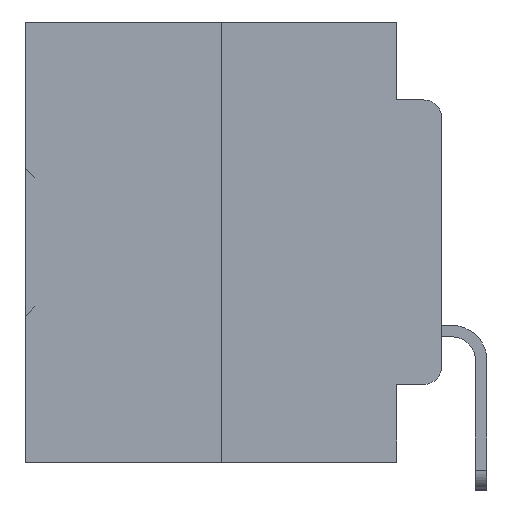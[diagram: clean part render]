
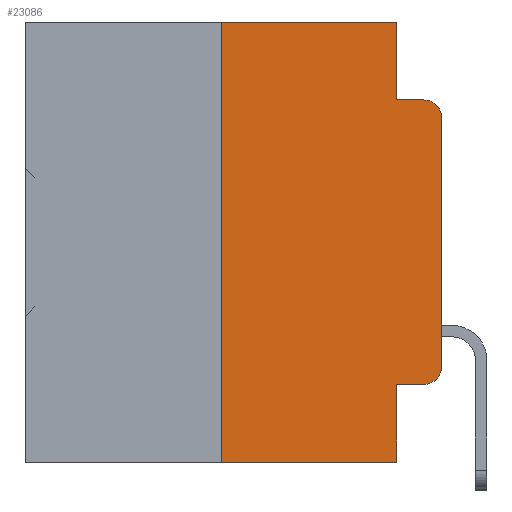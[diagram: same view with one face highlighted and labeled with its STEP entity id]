
A CAD part, left-side view. The second image highlights one B-rep face of the part: STEP entity #23086.
In plain terms, the highlighted planar face has unit normal (-1, 0, 0).
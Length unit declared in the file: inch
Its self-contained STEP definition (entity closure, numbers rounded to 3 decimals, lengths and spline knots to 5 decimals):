
#626 = DIRECTION ( 'NONE',  ( 0., 0., -1. ) ) ;
#1160 = CARTESIAN_POINT ( 'NONE',  ( 0., 0.051, -0.0885 ) ) ;
#1191 = DIRECTION ( 'NONE',  ( 0., -1., 0. ) ) ;
#1412 = ORIENTED_EDGE ( 'NONE', *, *, #22082, .F. ) ;
#1451 = ORIENTED_EDGE ( 'NONE', *, *, #6704, .T. ) ;
#1999 = ORIENTED_EDGE ( 'NONE', *, *, #4632, .T. ) ;
#2195 = ORIENTED_EDGE ( 'NONE', *, *, #2540, .F. ) ;
#2540 = EDGE_CURVE ( 'NONE', #16246, #21346, #27985, .T. ) ;
#3675 = VECTOR ( 'NONE', #13555, 39.37008 ) ;
#4481 = VECTOR ( 'NONE', #35738, 39.37008 ) ;
#4632 = EDGE_CURVE ( 'NONE', #16246, #25232, #21026, .T. ) ;
#5987 = CARTESIAN_POINT ( 'NONE',  ( 0., 0.051, -0.0885 ) ) ;
#6345 = ORIENTED_EDGE ( 'NONE', *, *, #34765, .F. ) ;
#6704 = EDGE_CURVE ( 'NONE', #25232, #14357, #8270, .T. ) ;
#8270 = CIRCLE ( 'NONE', #35639, 0.02 ) ;
#8924 = CARTESIAN_POINT ( 'NONE',  ( 0., 0.25, 0. ) ) ;
#9318 = AXIS2_PLACEMENT_3D ( 'NONE', #10441, #10568, #30804 ) ;
#9824 = CARTESIAN_POINT ( 'NONE',  ( 0., 0., -0.3915 ) ) ;
#10441 = CARTESIAN_POINT ( 'NONE',  ( 0., 0.473, 0. ) ) ;
#10568 = DIRECTION ( 'NONE',  ( 1., 0., 0. ) ) ;
#10607 = VERTEX_POINT ( 'NONE', #23813 ) ;
#10958 = LINE ( 'NONE', #8924, #32226 ) ;
#11064 = LINE ( 'NONE', #36434, #24773 ) ;
#11649 = ORIENTED_EDGE ( 'NONE', *, *, #23069, .T. ) ;
#11837 = LINE ( 'NONE', #1160, #3675 ) ;
#11962 = DIRECTION ( 'NONE',  ( 0., -1., 0. ) ) ;
#12169 = CARTESIAN_POINT ( 'NONE',  ( 0., 0.473, 0. ) ) ;
#13006 = VECTOR ( 'NONE', #626, 39.37008 ) ;
#13555 = DIRECTION ( 'NONE',  ( 0., -1., 0. ) ) ;
#13942 = CARTESIAN_POINT ( 'NONE',  ( 0., 0.051, -0.4115 ) ) ;
#13976 = ORIENTED_EDGE ( 'NONE', *, *, #21432, .T. ) ;
#14116 = ORIENTED_EDGE ( 'NONE', *, *, #25229, .F. ) ;
#14357 = VERTEX_POINT ( 'NONE', #9824 ) ;
#14904 = CIRCLE ( 'NONE', #19058, 0.02 ) ;
#15315 = VECTOR ( 'NONE', #21055, 39.37008 ) ;
#15447 = DIRECTION ( 'NONE',  ( -1., 0., 0. ) ) ;
#16090 = CARTESIAN_POINT ( 'NONE',  ( 0., 0.25, -0.5 ) ) ;
#16244 = LINE ( 'NONE', #12169, #15315 ) ;
#16246 = VERTEX_POINT ( 'NONE', #13942 ) ;
#16647 = ORIENTED_EDGE ( 'NONE', *, *, #19540, .T. ) ;
#17159 = FACE_OUTER_BOUND ( 'NONE', #35326, .T. ) ;
#17378 = ORIENTED_EDGE ( 'NONE', *, *, #32853, .F. ) ;
#17416 = CARTESIAN_POINT ( 'NONE',  ( 0., 0.02, -0.0885 ) ) ;
#17873 = CARTESIAN_POINT ( 'NONE',  ( 0., 0.25, 0. ) ) ;
#18340 = CARTESIAN_POINT ( 'NONE',  ( 0., 0.02, -0.1085 ) ) ;
#19058 = AXIS2_PLACEMENT_3D ( 'NONE', #18340, #37936, #21225 ) ;
#19540 = EDGE_CURVE ( 'NONE', #14357, #10607, #35267, .T. ) ;
#20838 = LINE ( 'NONE', #33101, #13006 ) ;
#21026 = LINE ( 'NONE', #32145, #27666 ) ;
#21055 = DIRECTION ( 'NONE',  ( 0., -1., 0. ) ) ;
#21064 = VECTOR ( 'NONE', #26533, 39.37008 ) ;
#21225 = DIRECTION ( 'NONE',  ( 0., 0., -1. ) ) ;
#21346 = VERTEX_POINT ( 'NONE', #23585 ) ;
#21432 = EDGE_CURVE ( 'NONE', #10607, #27929, #14904, .T. ) ;
#22082 = EDGE_CURVE ( 'NONE', #28594, #37106, #16244, .T. ) ;
#23069 = EDGE_CURVE ( 'NONE', #32886, #21346, #11064, .T. ) ;
#23086 = ADVANCED_FACE ( 'NONE', ( #17159 ), #27964, .F. ) ;
#23585 = CARTESIAN_POINT ( 'NONE',  ( 0., 0.051, -0.5 ) ) ;
#23696 = CARTESIAN_POINT ( 'NONE',  ( 0., 0., 0. ) ) ;
#23813 = CARTESIAN_POINT ( 'NONE',  ( 0., 0., -0.1085 ) ) ;
#24773 = VECTOR ( 'NONE', #1191, 39.37008 ) ;
#25229 = EDGE_CURVE ( 'NONE', #30576, #27929, #11837, .T. ) ;
#25232 = VERTEX_POINT ( 'NONE', #27943 ) ;
#26533 = DIRECTION ( 'NONE',  ( 0., 0., 1. ) ) ;
#27666 = VECTOR ( 'NONE', #11962, 39.37008 ) ;
#27929 = VERTEX_POINT ( 'NONE', #17416 ) ;
#27943 = CARTESIAN_POINT ( 'NONE',  ( 0., 0.02, -0.4115 ) ) ;
#27964 = PLANE ( 'NONE',  #9318 ) ;
#27985 = LINE ( 'NONE', #30005, #4481 ) ;
#28594 = VERTEX_POINT ( 'NONE', #17873 ) ;
#30005 = CARTESIAN_POINT ( 'NONE',  ( 0., 0.051, 0. ) ) ;
#30576 = VERTEX_POINT ( 'NONE', #5987 ) ;
#30804 = DIRECTION ( 'NONE',  ( 0., 0., -1. ) ) ;
#32145 = CARTESIAN_POINT ( 'NONE',  ( 0., 0.051, -0.4115 ) ) ;
#32226 = VECTOR ( 'NONE', #37849, 39.37008 ) ;
#32604 = CARTESIAN_POINT ( 'NONE',  ( 0., 0.02, -0.3915 ) ) ;
#32853 = EDGE_CURVE ( 'NONE', #37106, #30576, #20838, .T. ) ;
#32886 = VERTEX_POINT ( 'NONE', #16090 ) ;
#33101 = CARTESIAN_POINT ( 'NONE',  ( 0., 0.051, 0. ) ) ;
#34351 = CARTESIAN_POINT ( 'NONE',  ( 0., 0.051, 0. ) ) ;
#34765 = EDGE_CURVE ( 'NONE', #32886, #28594, #10958, .T. ) ;
#35267 = LINE ( 'NONE', #23696, #21064 ) ;
#35326 = EDGE_LOOP ( 'NONE', ( #16647, #13976, #14116, #17378, #1412, #6345, #11649, #2195, #1999, #1451 ) ) ;
#35456 = DIRECTION ( 'NONE',  ( 0., 0., -1. ) ) ;
#35639 = AXIS2_PLACEMENT_3D ( 'NONE', #32604, #15447, #35456 ) ;
#35738 = DIRECTION ( 'NONE',  ( 0., 0., -1. ) ) ;
#36434 = CARTESIAN_POINT ( 'NONE',  ( 0., 0.473, -0.5 ) ) ;
#37106 = VERTEX_POINT ( 'NONE', #34351 ) ;
#37849 = DIRECTION ( 'NONE',  ( 0., 0., 1. ) ) ;
#37936 = DIRECTION ( 'NONE',  ( -1., 0., 0. ) ) ;
